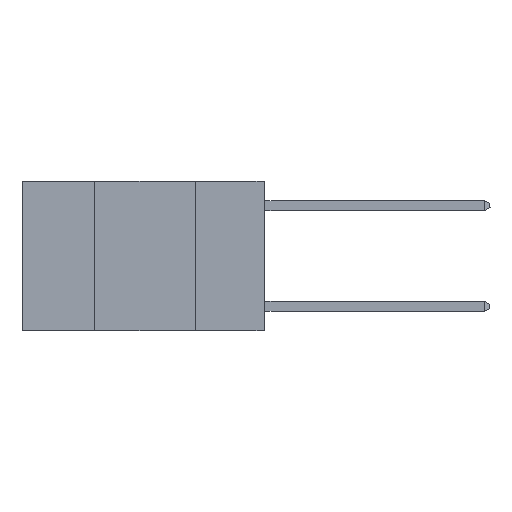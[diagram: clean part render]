
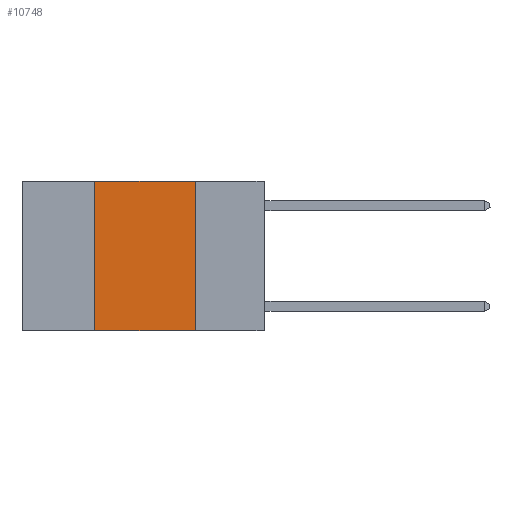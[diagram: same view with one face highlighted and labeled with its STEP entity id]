
A CAD part, left-side view. The second image highlights one B-rep face of the part: STEP entity #10748.
In plain terms, the highlighted planar face has unit normal (-1, 0, 0).
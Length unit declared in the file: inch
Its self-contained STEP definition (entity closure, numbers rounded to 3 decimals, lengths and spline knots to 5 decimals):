
#137 = VECTOR ( 'NONE', #4305, 39.37008 ) ;
#1350 = DIRECTION ( 'NONE',  ( 0., -1., 0. ) ) ;
#1437 = CARTESIAN_POINT ( 'NONE',  ( 0., 0.42, 0. ) ) ;
#1821 = VERTEX_POINT ( 'NONE', #4286 ) ;
#2008 = CARTESIAN_POINT ( 'NONE',  ( 0., 0.17, 0. ) ) ;
#2086 = VECTOR ( 'NONE', #1350, 39.37008 ) ;
#2171 = ORIENTED_EDGE ( 'NONE', *, *, #8061, .F. ) ;
#2342 = FACE_OUTER_BOUND ( 'NONE', #10126, .T. ) ;
#3068 = CARTESIAN_POINT ( 'NONE',  ( 0., 0.17, -0.37 ) ) ;
#3206 = LINE ( 'NONE', #11062, #9352 ) ;
#3452 = PLANE ( 'NONE',  #6325 ) ;
#3895 = ORIENTED_EDGE ( 'NONE', *, *, #14693, .F. ) ;
#3978 = VECTOR ( 'NONE', #4907, 39.37008 ) ;
#4286 = CARTESIAN_POINT ( 'NONE',  ( 0., 0.42, -0.37 ) ) ;
#4305 = DIRECTION ( 'NONE',  ( 0., 0., 1. ) ) ;
#4595 = ORIENTED_EDGE ( 'NONE', *, *, #12839, .T. ) ;
#4684 = DIRECTION ( 'NONE',  ( 1., 0., 0. ) ) ;
#4907 = DIRECTION ( 'NONE',  ( 0., 0., -1. ) ) ;
#4958 = VERTEX_POINT ( 'NONE', #1437 ) ;
#6271 = LINE ( 'NONE', #11677, #137 ) ;
#6325 = AXIS2_PLACEMENT_3D ( 'NONE', #10797, #4684, #13247 ) ;
#6507 = VERTEX_POINT ( 'NONE', #3068 ) ;
#7255 = LINE ( 'NONE', #13432, #3978 ) ;
#8061 = EDGE_CURVE ( 'NONE', #4958, #12000, #3206, .T. ) ;
#9352 = VECTOR ( 'NONE', #12360, 39.37008 ) ;
#10126 = EDGE_LOOP ( 'NONE', ( #3895, #2171, #15044, #4595 ) ) ;
#10748 = ADVANCED_FACE ( 'NONE', ( #2342 ), #3452, .F. ) ;
#10797 = CARTESIAN_POINT ( 'NONE',  ( 0., 0.6, 0. ) ) ;
#11062 = CARTESIAN_POINT ( 'NONE',  ( 0., 0.6, 0. ) ) ;
#11677 = CARTESIAN_POINT ( 'NONE',  ( 0., 0.42, 0. ) ) ;
#11899 = LINE ( 'NONE', #14762, #2086 ) ;
#12000 = VERTEX_POINT ( 'NONE', #2008 ) ;
#12360 = DIRECTION ( 'NONE',  ( 0., -1., 0. ) ) ;
#12839 = EDGE_CURVE ( 'NONE', #1821, #6507, #11899, .T. ) ;
#13247 = DIRECTION ( 'NONE',  ( 0., 0., -1. ) ) ;
#13432 = CARTESIAN_POINT ( 'NONE',  ( 0., 0.17, 0. ) ) ;
#14693 = EDGE_CURVE ( 'NONE', #12000, #6507, #7255, .T. ) ;
#14762 = CARTESIAN_POINT ( 'NONE',  ( 0., 0.6, -0.37 ) ) ;
#15002 = EDGE_CURVE ( 'NONE', #1821, #4958, #6271, .T. ) ;
#15044 = ORIENTED_EDGE ( 'NONE', *, *, #15002, .F. ) ;
